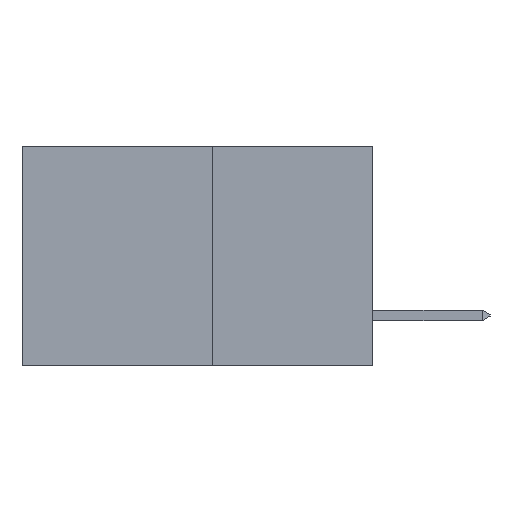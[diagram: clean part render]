
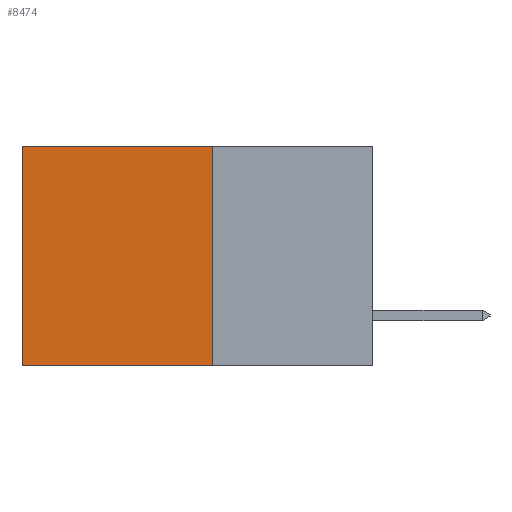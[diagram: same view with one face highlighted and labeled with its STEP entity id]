
A CAD part, left-side view. The second image highlights one B-rep face of the part: STEP entity #8474.
In plain terms, the highlighted planar face has unit normal (-1, 0, 0).
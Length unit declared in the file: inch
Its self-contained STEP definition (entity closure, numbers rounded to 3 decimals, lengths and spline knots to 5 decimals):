
#391 = VECTOR ( 'NONE', #424, 39.37008 ) ;
#394 = CARTESIAN_POINT ( 'NONE',  ( 0.277, 0.59, -0.37 ) ) ;
#424 = DIRECTION ( 'NONE',  ( 0., 0., -1. ) ) ;
#670 = VERTEX_POINT ( 'NONE', #6249 ) ;
#1916 = EDGE_CURVE ( 'NONE', #8940, #670, #12738, .T. ) ;
#2045 = CARTESIAN_POINT ( 'NONE',  ( 0.277, 0.27, -0.37 ) ) ;
#3418 = ORIENTED_EDGE ( 'NONE', *, *, #11125, .F. ) ;
#4358 = CARTESIAN_POINT ( 'NONE',  ( 0.277, 0.27, -0.37 ) ) ;
#4407 = DIRECTION ( 'NONE',  ( 1., 0., 0. ) ) ;
#4455 = AXIS2_PLACEMENT_3D ( 'NONE', #4358, #4407, #11886 ) ;
#5005 = VERTEX_POINT ( 'NONE', #8628 ) ;
#5036 = CARTESIAN_POINT ( 'NONE',  ( 0.277, 0.59, -0.37 ) ) ;
#5090 = DIRECTION ( 'NONE',  ( 0., 1., 0. ) ) ;
#5745 = EDGE_LOOP ( 'NONE', ( #12596, #3418, #10092, #6987 ) ) ;
#6249 = CARTESIAN_POINT ( 'NONE',  ( 0.277, 0.59, 0. ) ) ;
#6310 = EDGE_CURVE ( 'NONE', #670, #7663, #6443, .T. ) ;
#6443 = LINE ( 'NONE', #394, #391 ) ;
#6987 = ORIENTED_EDGE ( 'NONE', *, *, #1916, .T. ) ;
#7149 = EDGE_CURVE ( 'NONE', #8940, #5005, #9952, .T. ) ;
#7278 = CARTESIAN_POINT ( 'NONE',  ( 0.277, 0.27, 0. ) ) ;
#7663 = VERTEX_POINT ( 'NONE', #5036 ) ;
#7941 = LINE ( 'NONE', #10487, #13570 ) ;
#8474 = ADVANCED_FACE ( 'NONE', ( #10722 ), #8714, .F. ) ;
#8628 = CARTESIAN_POINT ( 'NONE',  ( 0.277, 0.27, -0.37 ) ) ;
#8714 = PLANE ( 'NONE',  #4455 ) ;
#8940 = VERTEX_POINT ( 'NONE', #9491 ) ;
#9292 = VECTOR ( 'NONE', #10466, 39.37008 ) ;
#9491 = CARTESIAN_POINT ( 'NONE',  ( 0.277, 0.27, 0. ) ) ;
#9952 = LINE ( 'NONE', #2045, #12399 ) ;
#10092 = ORIENTED_EDGE ( 'NONE', *, *, #7149, .F. ) ;
#10466 = DIRECTION ( 'NONE',  ( 0., 1., 0. ) ) ;
#10487 = CARTESIAN_POINT ( 'NONE',  ( 0.277, 0.27, -0.37 ) ) ;
#10634 = DIRECTION ( 'NONE',  ( 0., 0., -1. ) ) ;
#10722 = FACE_OUTER_BOUND ( 'NONE', #5745, .T. ) ;
#11125 = EDGE_CURVE ( 'NONE', #5005, #7663, #7941, .T. ) ;
#11886 = DIRECTION ( 'NONE',  ( 0., 0., -1. ) ) ;
#12399 = VECTOR ( 'NONE', #10634, 39.37008 ) ;
#12596 = ORIENTED_EDGE ( 'NONE', *, *, #6310, .T. ) ;
#12738 = LINE ( 'NONE', #7278, #9292 ) ;
#13570 = VECTOR ( 'NONE', #5090, 39.37008 ) ;
